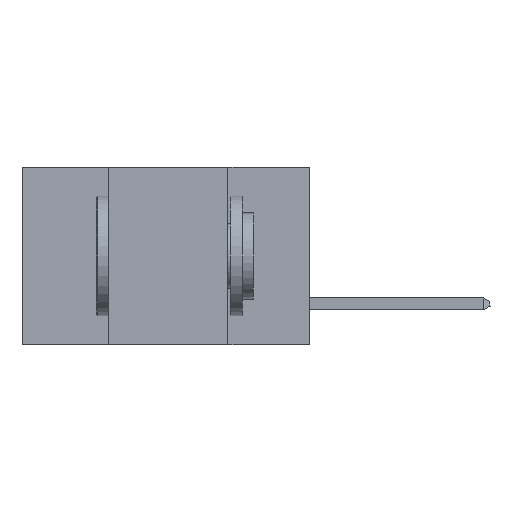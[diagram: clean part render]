
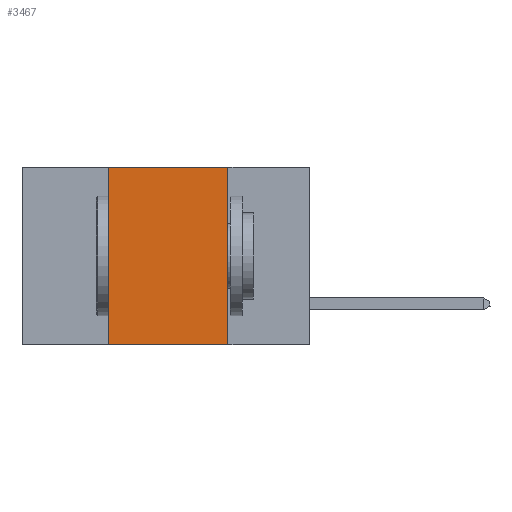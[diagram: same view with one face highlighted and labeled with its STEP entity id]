
A CAD part, left-side view. The second image highlights one B-rep face of the part: STEP entity #3467.
In plain terms, the highlighted planar face has unit normal (-1, 0, 0).
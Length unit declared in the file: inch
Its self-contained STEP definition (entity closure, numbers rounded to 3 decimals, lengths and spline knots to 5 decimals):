
#52 = AXIS2_PLACEMENT_3D ( 'NONE', #10907, #5525, #5330 ) ;
#535 = VERTEX_POINT ( 'NONE', #769 ) ;
#769 = CARTESIAN_POINT ( 'NONE',  ( 0., 0.17, -0.37 ) ) ;
#2520 = LINE ( 'NONE', #8250, #6020 ) ;
#3229 = EDGE_LOOP ( 'NONE', ( #8251, #5217, #3896, #6824 ) ) ;
#3467 = ADVANCED_FACE ( 'NONE', ( #9939 ), #12982, .F. ) ;
#3472 = VECTOR ( 'NONE', #11796, 39.37008 ) ;
#3896 = ORIENTED_EDGE ( 'NONE', *, *, #6651, .F. ) ;
#4038 = VERTEX_POINT ( 'NONE', #4497 ) ;
#4497 = CARTESIAN_POINT ( 'NONE',  ( 0., 0.42, -0.37 ) ) ;
#5217 = ORIENTED_EDGE ( 'NONE', *, *, #8671, .F. ) ;
#5235 = CARTESIAN_POINT ( 'NONE',  ( 0., 0.6, -0.37 ) ) ;
#5317 = VERTEX_POINT ( 'NONE', #11615 ) ;
#5330 = DIRECTION ( 'NONE',  ( 0., 0., -1. ) ) ;
#5525 = DIRECTION ( 'NONE',  ( 1., 0., 0. ) ) ;
#6020 = VECTOR ( 'NONE', #13738, 39.37008 ) ;
#6286 = LINE ( 'NONE', #5235, #3472 ) ;
#6358 = LINE ( 'NONE', #13090, #8568 ) ;
#6524 = DIRECTION ( 'NONE',  ( 0., 0., -1. ) ) ;
#6651 = EDGE_CURVE ( 'NONE', #4038, #5317, #10861, .T. ) ;
#6824 = ORIENTED_EDGE ( 'NONE', *, *, #11220, .T. ) ;
#8250 = CARTESIAN_POINT ( 'NONE',  ( 0., 0.6, 0. ) ) ;
#8251 = ORIENTED_EDGE ( 'NONE', *, *, #9309, .F. ) ;
#8568 = VECTOR ( 'NONE', #6524, 39.37008 ) ;
#8671 = EDGE_CURVE ( 'NONE', #5317, #12890, #2520, .T. ) ;
#9309 = EDGE_CURVE ( 'NONE', #12890, #535, #6358, .T. ) ;
#9939 = FACE_OUTER_BOUND ( 'NONE', #3229, .T. ) ;
#10861 = LINE ( 'NONE', #11270, #13385 ) ;
#10907 = CARTESIAN_POINT ( 'NONE',  ( 0., 0.6, 0. ) ) ;
#11220 = EDGE_CURVE ( 'NONE', #4038, #535, #6286, .T. ) ;
#11270 = CARTESIAN_POINT ( 'NONE',  ( 0., 0.42, 0. ) ) ;
#11615 = CARTESIAN_POINT ( 'NONE',  ( 0., 0.42, 0. ) ) ;
#11796 = DIRECTION ( 'NONE',  ( 0., -1., 0. ) ) ;
#12890 = VERTEX_POINT ( 'NONE', #13063 ) ;
#12982 = PLANE ( 'NONE',  #52 ) ;
#13029 = DIRECTION ( 'NONE',  ( 0., 0., 1. ) ) ;
#13063 = CARTESIAN_POINT ( 'NONE',  ( 0., 0.17, 0. ) ) ;
#13090 = CARTESIAN_POINT ( 'NONE',  ( 0., 0.17, 0. ) ) ;
#13385 = VECTOR ( 'NONE', #13029, 39.37008 ) ;
#13738 = DIRECTION ( 'NONE',  ( 0., -1., 0. ) ) ;
